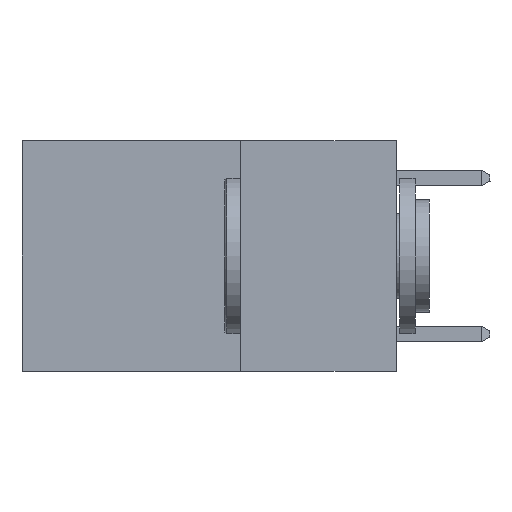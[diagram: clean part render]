
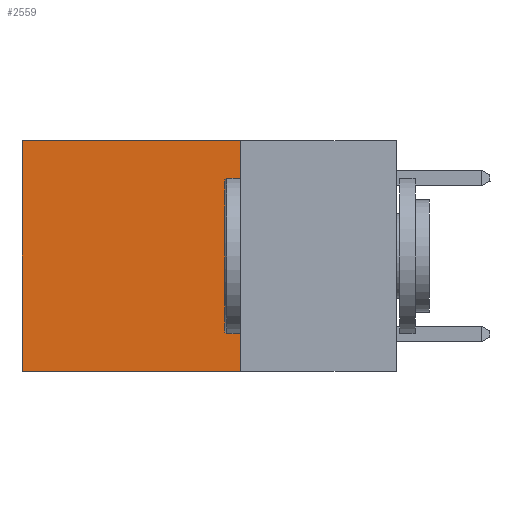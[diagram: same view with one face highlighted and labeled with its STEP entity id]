
A CAD part, left-side view. The second image highlights one B-rep face of the part: STEP entity #2559.
In plain terms, the highlighted planar face has unit normal (-1, 0, 0).
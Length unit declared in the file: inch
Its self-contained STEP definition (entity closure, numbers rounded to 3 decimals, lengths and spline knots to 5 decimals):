
#89 = DIRECTION ( 'NONE',  ( 0., 0., -1. ) ) ;
#2417 = DIRECTION ( 'NONE',  ( 0., 1., 0. ) ) ;
#2559 = ADVANCED_FACE ( 'NONE', ( #14521 ), #9319, .F. ) ;
#2669 = LINE ( 'NONE', #11071, #10679 ) ;
#2801 = EDGE_CURVE ( 'NONE', #15015, #7114, #7560, .T. ) ;
#3247 = CARTESIAN_POINT ( 'NONE',  ( 0.2625, 0.25, 0. ) ) ;
#3595 = ORIENTED_EDGE ( 'NONE', *, *, #13565, .F. ) ;
#3742 = CARTESIAN_POINT ( 'NONE',  ( 0.2625, 0.25, 0. ) ) ;
#3774 = DIRECTION ( 'NONE',  ( 0., 1., 0. ) ) ;
#3956 = CARTESIAN_POINT ( 'NONE',  ( 0.2625, 0.6, 0. ) ) ;
#4411 = ORIENTED_EDGE ( 'NONE', *, *, #9651, .T. ) ;
#5785 = VECTOR ( 'NONE', #2417, 39.37008 ) ;
#5996 = VECTOR ( 'NONE', #3774, 39.37008 ) ;
#6410 = CARTESIAN_POINT ( 'NONE',  ( 0.2625, 0.25, 0. ) ) ;
#7114 = VERTEX_POINT ( 'NONE', #3956 ) ;
#7358 = DIRECTION ( 'NONE',  ( 0., 0., -1. ) ) ;
#7560 = LINE ( 'NONE', #3742, #5785 ) ;
#7583 = ORIENTED_EDGE ( 'NONE', *, *, #2801, .T. ) ;
#8014 = CARTESIAN_POINT ( 'NONE',  ( 0.2625, 0.25, 0. ) ) ;
#8264 = CARTESIAN_POINT ( 'NONE',  ( 0.2625, 0.25, -0.37 ) ) ;
#9111 = CARTESIAN_POINT ( 'NONE',  ( 0.2625, 0.25, -0.37 ) ) ;
#9180 = VERTEX_POINT ( 'NONE', #12693 ) ;
#9319 = PLANE ( 'NONE',  #15458 ) ;
#9651 = EDGE_CURVE ( 'NONE', #7114, #9180, #2669, .T. ) ;
#10457 = EDGE_LOOP ( 'NONE', ( #4411, #14280, #3595, #7583 ) ) ;
#10624 = DIRECTION ( 'NONE',  ( 0., 0., -1. ) ) ;
#10679 = VECTOR ( 'NONE', #7358, 39.37008 ) ;
#10994 = EDGE_CURVE ( 'NONE', #12619, #9180, #15880, .T. ) ;
#11071 = CARTESIAN_POINT ( 'NONE',  ( 0.2625, 0.6, 0. ) ) ;
#11304 = VECTOR ( 'NONE', #89, 39.37008 ) ;
#12619 = VERTEX_POINT ( 'NONE', #8264 ) ;
#12643 = LINE ( 'NONE', #8014, #11304 ) ;
#12693 = CARTESIAN_POINT ( 'NONE',  ( 0.2625, 0.6, -0.37 ) ) ;
#13192 = DIRECTION ( 'NONE',  ( 1., 0., 0. ) ) ;
#13565 = EDGE_CURVE ( 'NONE', #15015, #12619, #12643, .T. ) ;
#14280 = ORIENTED_EDGE ( 'NONE', *, *, #10994, .F. ) ;
#14521 = FACE_OUTER_BOUND ( 'NONE', #10457, .T. ) ;
#15015 = VERTEX_POINT ( 'NONE', #6410 ) ;
#15458 = AXIS2_PLACEMENT_3D ( 'NONE', #3247, #13192, #10624 ) ;
#15880 = LINE ( 'NONE', #9111, #5996 ) ;
